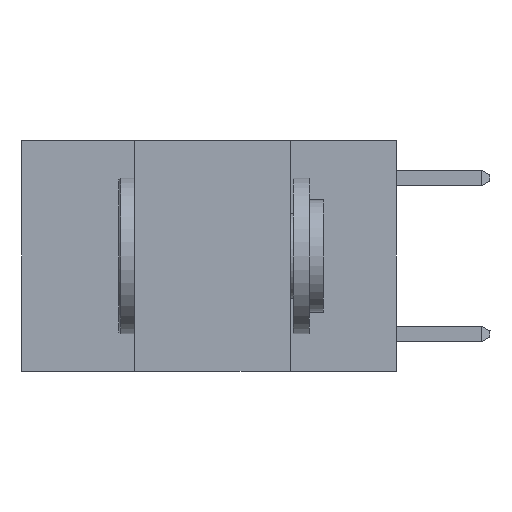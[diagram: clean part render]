
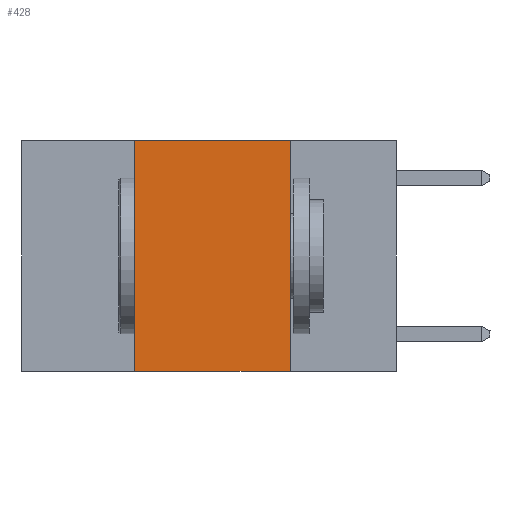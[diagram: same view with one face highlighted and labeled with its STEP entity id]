
A CAD part, left-side view. The second image highlights one B-rep face of the part: STEP entity #428.
In plain terms, the highlighted planar face has unit normal (-1, 0, 0).
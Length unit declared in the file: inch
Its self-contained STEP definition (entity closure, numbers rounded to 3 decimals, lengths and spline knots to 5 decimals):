
#88 = VERTEX_POINT ( 'NONE', #10583 ) ;
#364 = DIRECTION ( 'NONE',  ( 0., 0., 1. ) ) ;
#428 = ADVANCED_FACE ( 'NONE', ( #2887 ), #2353, .F. ) ;
#439 = ORIENTED_EDGE ( 'NONE', *, *, #2407, .T. ) ;
#1286 = CARTESIAN_POINT ( 'NONE',  ( 0., 0.6, -0.37 ) ) ;
#1524 = CARTESIAN_POINT ( 'NONE',  ( 0., 0.42, 0. ) ) ;
#1987 = DIRECTION ( 'NONE',  ( 0., 0., -1. ) ) ;
#2353 = PLANE ( 'NONE',  #11872 ) ;
#2407 = EDGE_CURVE ( 'NONE', #7608, #88, #3020, .T. ) ;
#2582 = DIRECTION ( 'NONE',  ( 1., 0., 0. ) ) ;
#2836 = ORIENTED_EDGE ( 'NONE', *, *, #6936, .F. ) ;
#2887 = FACE_OUTER_BOUND ( 'NONE', #5867, .T. ) ;
#3020 = LINE ( 'NONE', #1286, #10133 ) ;
#3288 = CARTESIAN_POINT ( 'NONE',  ( 0., 0.42, -0.37 ) ) ;
#4009 = ORIENTED_EDGE ( 'NONE', *, *, #9326, .F. ) ;
#4075 = VECTOR ( 'NONE', #8033, 39.37008 ) ;
#5033 = VERTEX_POINT ( 'NONE', #7545 ) ;
#5332 = VECTOR ( 'NONE', #8933, 39.37008 ) ;
#5867 = EDGE_LOOP ( 'NONE', ( #11074, #2836, #4009, #439 ) ) ;
#5934 = VERTEX_POINT ( 'NONE', #1524 ) ;
#6936 = EDGE_CURVE ( 'NONE', #5934, #5033, #7842, .T. ) ;
#7138 = CARTESIAN_POINT ( 'NONE',  ( 0., 0.17, 0. ) ) ;
#7545 = CARTESIAN_POINT ( 'NONE',  ( 0., 0.17, 0. ) ) ;
#7608 = VERTEX_POINT ( 'NONE', #3288 ) ;
#7842 = LINE ( 'NONE', #10647, #5332 ) ;
#8033 = DIRECTION ( 'NONE',  ( 0., 0., -1. ) ) ;
#8933 = DIRECTION ( 'NONE',  ( 0., -1., 0. ) ) ;
#9226 = CARTESIAN_POINT ( 'NONE',  ( 0., 0.6, 0. ) ) ;
#9286 = LINE ( 'NONE', #7138, #4075 ) ;
#9298 = LINE ( 'NONE', #11621, #11583 ) ;
#9326 = EDGE_CURVE ( 'NONE', #7608, #5934, #9298, .T. ) ;
#10133 = VECTOR ( 'NONE', #11500, 39.37008 ) ;
#10483 = EDGE_CURVE ( 'NONE', #5033, #88, #9286, .T. ) ;
#10583 = CARTESIAN_POINT ( 'NONE',  ( 0., 0.17, -0.37 ) ) ;
#10647 = CARTESIAN_POINT ( 'NONE',  ( 0., 0.6, 0. ) ) ;
#11074 = ORIENTED_EDGE ( 'NONE', *, *, #10483, .F. ) ;
#11500 = DIRECTION ( 'NONE',  ( 0., -1., 0. ) ) ;
#11583 = VECTOR ( 'NONE', #364, 39.37008 ) ;
#11621 = CARTESIAN_POINT ( 'NONE',  ( 0., 0.42, 0. ) ) ;
#11872 = AXIS2_PLACEMENT_3D ( 'NONE', #9226, #2582, #1987 ) ;
